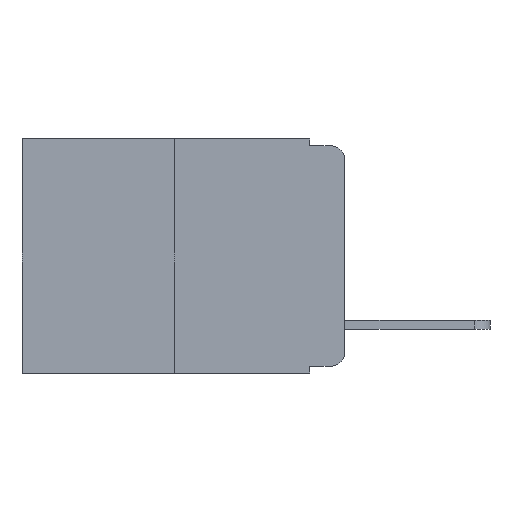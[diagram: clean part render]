
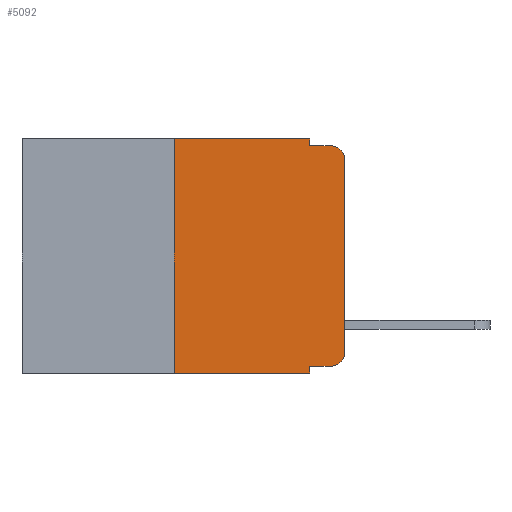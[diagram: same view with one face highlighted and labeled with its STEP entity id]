
A CAD part, left-side view. The second image highlights one B-rep face of the part: STEP entity #5092.
In plain terms, the highlighted planar face has unit normal (-1, 0, 0).
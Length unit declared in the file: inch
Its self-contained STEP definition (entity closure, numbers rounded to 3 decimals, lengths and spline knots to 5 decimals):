
#27 = DIRECTION ( 'NONE',  ( 0., 0., -1. ) ) ;
#282 = CARTESIAN_POINT ( 'NONE',  ( 0., 0.473, 0. ) ) ;
#365 = CARTESIAN_POINT ( 'NONE',  ( 0., 0.051, 0. ) ) ;
#432 = AXIS2_PLACEMENT_3D ( 'NONE', #1491, #10882, #5917 ) ;
#469 = EDGE_CURVE ( 'NONE', #1765, #3396, #9522, .T. ) ;
#532 = LINE ( 'NONE', #365, #5412 ) ;
#1188 = DIRECTION ( 'NONE',  ( -1., 0., 0. ) ) ;
#1208 = CARTESIAN_POINT ( 'NONE',  ( 0., 0.051, -0.01 ) ) ;
#1245 = VECTOR ( 'NONE', #6186, 39.37008 ) ;
#1278 = DIRECTION ( 'NONE',  ( 1., 0., 0. ) ) ;
#1440 = CARTESIAN_POINT ( 'NONE',  ( 0., 0.25, 0. ) ) ;
#1491 = CARTESIAN_POINT ( 'NONE',  ( 0., 0.02, -0.313 ) ) ;
#1765 = VERTEX_POINT ( 'NONE', #10051 ) ;
#2017 = LINE ( 'NONE', #1440, #6044 ) ;
#2160 = DIRECTION ( 'NONE',  ( 0., 0., -1. ) ) ;
#2265 = EDGE_CURVE ( 'NONE', #6543, #6902, #6584, .T. ) ;
#2289 = VECTOR ( 'NONE', #10694, 39.37008 ) ;
#2291 = VERTEX_POINT ( 'NONE', #6356 ) ;
#2503 = CARTESIAN_POINT ( 'NONE',  ( 0., 0., -0.03 ) ) ;
#2519 = EDGE_CURVE ( 'NONE', #2650, #6543, #532, .T. ) ;
#2587 = CARTESIAN_POINT ( 'NONE',  ( 0., 0.25, 0. ) ) ;
#2650 = VERTEX_POINT ( 'NONE', #8620 ) ;
#2737 = EDGE_CURVE ( 'NONE', #8946, #5047, #9608, .T. ) ;
#2767 = EDGE_CURVE ( 'NONE', #9089, #4870, #2017, .T. ) ;
#3323 = CIRCLE ( 'NONE', #9428, 0.02 ) ;
#3396 = VERTEX_POINT ( 'NONE', #2503 ) ;
#3452 = VECTOR ( 'NONE', #27, 39.37008 ) ;
#3485 = VECTOR ( 'NONE', #10588, 39.37008 ) ;
#3487 = CARTESIAN_POINT ( 'NONE',  ( 0., 0.25, -0.343 ) ) ;
#3626 = ORIENTED_EDGE ( 'NONE', *, *, #2519, .F. ) ;
#3744 = ORIENTED_EDGE ( 'NONE', *, *, #8563, .F. ) ;
#3831 = CIRCLE ( 'NONE', #432, 0.02 ) ;
#3887 = CARTESIAN_POINT ( 'NONE',  ( 0., 0.051, -0.333 ) ) ;
#4058 = EDGE_CURVE ( 'NONE', #8946, #2291, #9452, .T. ) ;
#4180 = DIRECTION ( 'NONE',  ( 0., 0., 1. ) ) ;
#4203 = EDGE_CURVE ( 'NONE', #3396, #6902, #3323, .T. ) ;
#4508 = ORIENTED_EDGE ( 'NONE', *, *, #5319, .T. ) ;
#4605 = LINE ( 'NONE', #8166, #2289 ) ;
#4619 = CARTESIAN_POINT ( 'NONE',  ( 0., 0.051, -0.333 ) ) ;
#4666 = CARTESIAN_POINT ( 'NONE',  ( 0., 0.051, -0.01 ) ) ;
#4810 = CARTESIAN_POINT ( 'NONE',  ( 0., 0., 0. ) ) ;
#4821 = ORIENTED_EDGE ( 'NONE', *, *, #4203, .T. ) ;
#4865 = ORIENTED_EDGE ( 'NONE', *, *, #2737, .T. ) ;
#4870 = VERTEX_POINT ( 'NONE', #2587 ) ;
#5047 = VERTEX_POINT ( 'NONE', #8050 ) ;
#5090 = CARTESIAN_POINT ( 'NONE',  ( 0., 0.051, 0. ) ) ;
#5092 = ADVANCED_FACE ( 'NONE', ( #9692 ), #6441, .F. ) ;
#5319 = EDGE_CURVE ( 'NONE', #5047, #1765, #3831, .T. ) ;
#5365 = ORIENTED_EDGE ( 'NONE', *, *, #6440, .T. ) ;
#5412 = VECTOR ( 'NONE', #5640, 39.37008 ) ;
#5577 = ORIENTED_EDGE ( 'NONE', *, *, #2767, .F. ) ;
#5601 = DIRECTION ( 'NONE',  ( 0., -1., 0. ) ) ;
#5634 = AXIS2_PLACEMENT_3D ( 'NONE', #282, #1278, #2160 ) ;
#5640 = DIRECTION ( 'NONE',  ( 0., 0., -1. ) ) ;
#5784 = VECTOR ( 'NONE', #5601, 39.37008 ) ;
#5917 = DIRECTION ( 'NONE',  ( 0., 0., -1. ) ) ;
#6044 = VECTOR ( 'NONE', #4180, 39.37008 ) ;
#6186 = DIRECTION ( 'NONE',  ( 0., -1., 0. ) ) ;
#6223 = CARTESIAN_POINT ( 'NONE',  ( 0., 0.473, -0.343 ) ) ;
#6356 = CARTESIAN_POINT ( 'NONE',  ( 0., 0.051, -0.343 ) ) ;
#6440 = EDGE_CURVE ( 'NONE', #9089, #2291, #6495, .T. ) ;
#6441 = PLANE ( 'NONE',  #5634 ) ;
#6495 = LINE ( 'NONE', #6223, #1245 ) ;
#6543 = VERTEX_POINT ( 'NONE', #1208 ) ;
#6584 = LINE ( 'NONE', #4666, #3485 ) ;
#6680 = ORIENTED_EDGE ( 'NONE', *, *, #469, .T. ) ;
#6902 = VERTEX_POINT ( 'NONE', #10980 ) ;
#7451 = ORIENTED_EDGE ( 'NONE', *, *, #2265, .F. ) ;
#7943 = DIRECTION ( 'NONE',  ( 0., 0., -1. ) ) ;
#8050 = CARTESIAN_POINT ( 'NONE',  ( 0., 0.02, -0.333 ) ) ;
#8166 = CARTESIAN_POINT ( 'NONE',  ( 0., 0.473, 0. ) ) ;
#8563 = EDGE_CURVE ( 'NONE', #4870, #2650, #4605, .T. ) ;
#8620 = CARTESIAN_POINT ( 'NONE',  ( 0., 0.051, 0. ) ) ;
#8721 = CARTESIAN_POINT ( 'NONE',  ( 0., 0.02, -0.03 ) ) ;
#8946 = VERTEX_POINT ( 'NONE', #4619 ) ;
#9089 = VERTEX_POINT ( 'NONE', #3487 ) ;
#9173 = ORIENTED_EDGE ( 'NONE', *, *, #4058, .F. ) ;
#9428 = AXIS2_PLACEMENT_3D ( 'NONE', #8721, #1188, #7943 ) ;
#9452 = LINE ( 'NONE', #5090, #3452 ) ;
#9522 = LINE ( 'NONE', #4810, #9779 ) ;
#9608 = LINE ( 'NONE', #3887, #5784 ) ;
#9692 = FACE_OUTER_BOUND ( 'NONE', #10078, .T. ) ;
#9779 = VECTOR ( 'NONE', #10729, 39.37008 ) ;
#10051 = CARTESIAN_POINT ( 'NONE',  ( 0., 0., -0.313 ) ) ;
#10078 = EDGE_LOOP ( 'NONE', ( #6680, #4821, #7451, #3626, #3744, #5577, #5365, #9173, #4865, #4508 ) ) ;
#10588 = DIRECTION ( 'NONE',  ( 0., -1., 0. ) ) ;
#10694 = DIRECTION ( 'NONE',  ( 0., -1., 0. ) ) ;
#10729 = DIRECTION ( 'NONE',  ( 0., 0., 1. ) ) ;
#10882 = DIRECTION ( 'NONE',  ( -1., 0., 0. ) ) ;
#10980 = CARTESIAN_POINT ( 'NONE',  ( 0., 0.02, -0.01 ) ) ;
